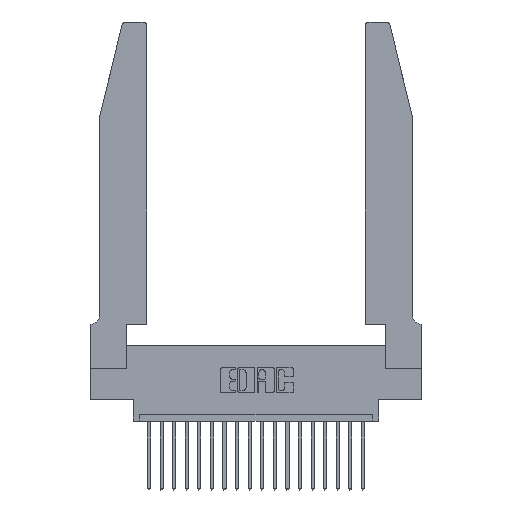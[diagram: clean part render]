
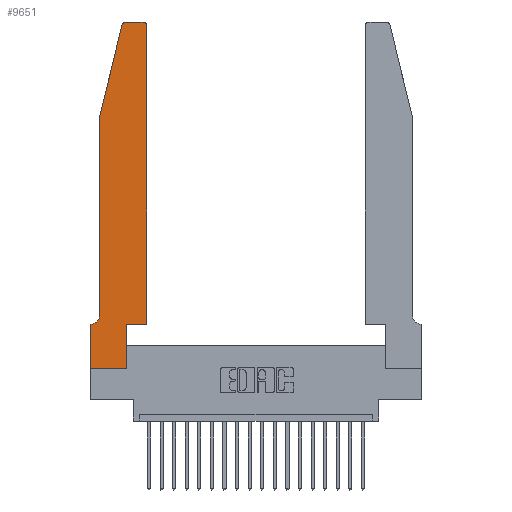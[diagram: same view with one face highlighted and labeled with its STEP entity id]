
A CAD part, top view. The second image highlights one B-rep face of the part: STEP entity #9651.
In plain terms, the highlighted planar face has unit normal (0, 0, 1).
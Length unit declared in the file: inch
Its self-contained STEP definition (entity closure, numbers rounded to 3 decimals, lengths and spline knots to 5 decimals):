
#288 = AXIS2_PLACEMENT_3D ( 'NONE', #14571, #17987, #19423 ) ;
#293 = EDGE_CURVE ( 'NONE', #20277, #7171, #17946, .T. ) ;
#461 = LINE ( 'NONE', #15051, #4130 ) ;
#670 = EDGE_CURVE ( 'NONE', #7828, #21630, #10143, .T. ) ;
#713 = CARTESIAN_POINT ( 'NONE',  ( 0.4505, 0.35, 0.37 ) ) ;
#761 = CIRCLE ( 'NONE', #5719, 0.07 ) ;
#1069 = VERTEX_POINT ( 'NONE', #11966 ) ;
#1301 = CARTESIAN_POINT ( 'NONE',  ( 0., 0., 0.37 ) ) ;
#1348 = CARTESIAN_POINT ( 'NONE',  ( 0.284, 2.75, 0.37 ) ) ;
#1577 = CARTESIAN_POINT ( 'NONE',  ( 0., 0.35, 0.37 ) ) ;
#1685 = CARTESIAN_POINT ( 'NONE',  ( 0.4505, 0.35, 0.37 ) ) ;
#1782 = VERTEX_POINT ( 'NONE', #5611 ) ;
#1983 = ORIENTED_EDGE ( 'NONE', *, *, #670, .T. ) ;
#2291 = DIRECTION ( 'NONE',  ( -1., 0., 0. ) ) ;
#2487 = CARTESIAN_POINT ( 'NONE',  ( 0.0055, 0.42, 0.37 ) ) ;
#3033 = EDGE_CURVE ( 'NONE', #17032, #6590, #10055, .T. ) ;
#3431 = DIRECTION ( 'NONE',  ( 1., 0., 0. ) ) ;
#3544 = VECTOR ( 'NONE', #13919, 39.37008 ) ;
#3933 = ORIENTED_EDGE ( 'NONE', *, *, #7599, .T. ) ;
#4130 = VECTOR ( 'NONE', #11509, 39.37008 ) ;
#4262 = PLANE ( 'NONE',  #12561 ) ;
#4383 = VECTOR ( 'NONE', #17783, 39.37008 ) ;
#4639 = LINE ( 'NONE', #16111, #4383 ) ;
#4814 = LINE ( 'NONE', #1301, #7707 ) ;
#5580 = EDGE_CURVE ( 'NONE', #17342, #1069, #461, .T. ) ;
#5611 = CARTESIAN_POINT ( 'NONE',  ( 0.0055, 0.35, 0.37 ) ) ;
#5719 = AXIS2_PLACEMENT_3D ( 'NONE', #2487, #16050, #9144 ) ;
#5727 = DIRECTION ( 'NONE',  ( -0.239, -0.971, 0. ) ) ;
#5855 = VERTEX_POINT ( 'NONE', #13804 ) ;
#5998 = CARTESIAN_POINT ( 'NONE',  ( 0., 0.35, 0.37 ) ) ;
#6560 = LINE ( 'NONE', #1685, #18860 ) ;
#6590 = VERTEX_POINT ( 'NONE', #12761 ) ;
#6754 = LINE ( 'NONE', #13740, #17758 ) ;
#7171 = VERTEX_POINT ( 'NONE', #8647 ) ;
#7323 = ORIENTED_EDGE ( 'NONE', *, *, #9769, .T. ) ;
#7378 = ORIENTED_EDGE ( 'NONE', *, *, #12603, .T. ) ;
#7599 = EDGE_CURVE ( 'NONE', #19247, #20277, #15832, .T. ) ;
#7707 = VECTOR ( 'NONE', #8265, 39.37008 ) ;
#7781 = DIRECTION ( 'NONE',  ( 0., 0., 1. ) ) ;
#7828 = VERTEX_POINT ( 'NONE', #9027 ) ;
#8265 = DIRECTION ( 'NONE',  ( 0., -1., 0. ) ) ;
#8363 = CARTESIAN_POINT ( 'NONE',  ( 0.4505, 2.72, 0.37 ) ) ;
#8647 = CARTESIAN_POINT ( 'NONE',  ( 0.4205, 2.75, 0.37 ) ) ;
#9027 = CARTESIAN_POINT ( 'NONE',  ( 0.2865, 0., 0.37 ) ) ;
#9144 = DIRECTION ( 'NONE',  ( -1., 0., 0. ) ) ;
#9236 = FACE_OUTER_BOUND ( 'NONE', #10103, .T. ) ;
#9341 = ORIENTED_EDGE ( 'NONE', *, *, #17902, .T. ) ;
#9502 = VERTEX_POINT ( 'NONE', #1577 ) ;
#9651 = ADVANCED_FACE ( 'NONE', ( #9236 ), #4262, .T. ) ;
#9769 = EDGE_CURVE ( 'NONE', #21630, #19247, #6560, .T. ) ;
#9951 = DIRECTION ( 'NONE',  ( 1., 0., 0. ) ) ;
#10055 = CIRCLE ( 'NONE', #14644, 0.03 ) ;
#10103 = EDGE_LOOP ( 'NONE', ( #7378, #12428, #14392, #12490, #14223, #9341, #21509, #19240, #1983, #7323, #3933, #20164 ) ) ;
#10143 = LINE ( 'NONE', #18862, #11951 ) ;
#11246 = CARTESIAN_POINT ( 'NONE',  ( 0.0755, 2., 0.37 ) ) ;
#11429 = EDGE_CURVE ( 'NONE', #5855, #7828, #6754, .T. ) ;
#11509 = DIRECTION ( 'NONE',  ( 0., -1., 0. ) ) ;
#11790 = LINE ( 'NONE', #17301, #14385 ) ;
#11951 = VECTOR ( 'NONE', #15661, 39.37008 ) ;
#11966 = CARTESIAN_POINT ( 'NONE',  ( 0.0755, 0.42, 0.37 ) ) ;
#12099 = CARTESIAN_POINT ( 'NONE',  ( 0.0755, 0.35, 0.37 ) ) ;
#12199 = CARTESIAN_POINT ( 'NONE',  ( 0.2865, 0.35, 0.37 ) ) ;
#12428 = ORIENTED_EDGE ( 'NONE', *, *, #3033, .T. ) ;
#12490 = ORIENTED_EDGE ( 'NONE', *, *, #5580, .T. ) ;
#12561 = AXIS2_PLACEMENT_3D ( 'NONE', #5998, #7781, #19444 ) ;
#12603 = EDGE_CURVE ( 'NONE', #7171, #17032, #4639, .T. ) ;
#12761 = CARTESIAN_POINT ( 'NONE',  ( 0.25487, 2.72718, 0.37 ) ) ;
#12982 = EDGE_CURVE ( 'NONE', #6590, #17342, #11790, .T. ) ;
#13295 = DIRECTION ( 'NONE',  ( 1., 0., 0. ) ) ;
#13317 = DIRECTION ( 'NONE',  ( 0., 0., 1. ) ) ;
#13740 = CARTESIAN_POINT ( 'NONE',  ( 0., 0., 0.37 ) ) ;
#13804 = CARTESIAN_POINT ( 'NONE',  ( 0., 0., 0.37 ) ) ;
#13919 = DIRECTION ( 'NONE',  ( 0., 1., 0. ) ) ;
#14223 = ORIENTED_EDGE ( 'NONE', *, *, #18622, .T. ) ;
#14385 = VECTOR ( 'NONE', #5727, 39.37008 ) ;
#14392 = ORIENTED_EDGE ( 'NONE', *, *, #12982, .T. ) ;
#14571 = CARTESIAN_POINT ( 'NONE',  ( 0.4205, 2.72, 0.37 ) ) ;
#14644 = AXIS2_PLACEMENT_3D ( 'NONE', #19749, #13317, #9951 ) ;
#15051 = CARTESIAN_POINT ( 'NONE',  ( 0.0755, 2., 0.37 ) ) ;
#15661 = DIRECTION ( 'NONE',  ( 0., 1., 0. ) ) ;
#15765 = EDGE_CURVE ( 'NONE', #9502, #5855, #4814, .T. ) ;
#15832 = LINE ( 'NONE', #15864, #3544 ) ;
#15864 = CARTESIAN_POINT ( 'NONE',  ( 0.4505, 0.35, 0.37 ) ) ;
#15969 = VECTOR ( 'NONE', #2291, 39.37008 ) ;
#16050 = DIRECTION ( 'NONE',  ( 0., 0., -1. ) ) ;
#16111 = CARTESIAN_POINT ( 'NONE',  ( 0.2605, 2.75, 0.37 ) ) ;
#17032 = VERTEX_POINT ( 'NONE', #1348 ) ;
#17301 = CARTESIAN_POINT ( 'NONE',  ( 0.0755, 2., 0.37 ) ) ;
#17342 = VERTEX_POINT ( 'NONE', #11246 ) ;
#17758 = VECTOR ( 'NONE', #13295, 39.37008 ) ;
#17783 = DIRECTION ( 'NONE',  ( -1., 0., 0. ) ) ;
#17902 = EDGE_CURVE ( 'NONE', #1782, #9502, #20404, .T. ) ;
#17946 = CIRCLE ( 'NONE', #288, 0.03 ) ;
#17987 = DIRECTION ( 'NONE',  ( 0., 0., 1. ) ) ;
#18622 = EDGE_CURVE ( 'NONE', #1069, #1782, #761, .T. ) ;
#18860 = VECTOR ( 'NONE', #3431, 39.37008 ) ;
#18862 = CARTESIAN_POINT ( 'NONE',  ( 0.2865, 0.35, 0.37 ) ) ;
#19240 = ORIENTED_EDGE ( 'NONE', *, *, #11429, .T. ) ;
#19247 = VERTEX_POINT ( 'NONE', #713 ) ;
#19423 = DIRECTION ( 'NONE',  ( 1., 0., 0. ) ) ;
#19444 = DIRECTION ( 'NONE',  ( 1., 0., 0. ) ) ;
#19749 = CARTESIAN_POINT ( 'NONE',  ( 0.284, 2.72, 0.37 ) ) ;
#20164 = ORIENTED_EDGE ( 'NONE', *, *, #293, .T. ) ;
#20277 = VERTEX_POINT ( 'NONE', #8363 ) ;
#20404 = LINE ( 'NONE', #12099, #15969 ) ;
#21509 = ORIENTED_EDGE ( 'NONE', *, *, #15765, .T. ) ;
#21630 = VERTEX_POINT ( 'NONE', #12199 ) ;
